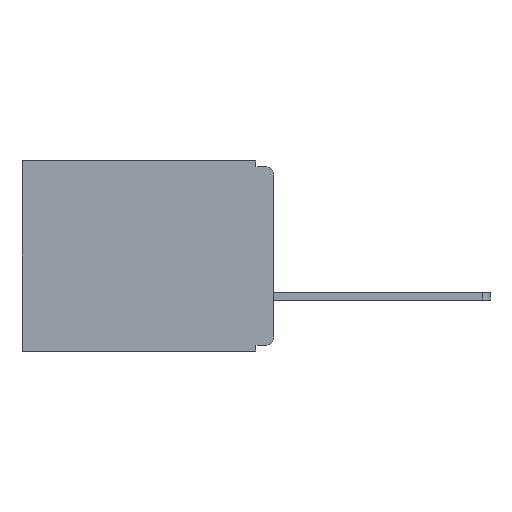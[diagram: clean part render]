
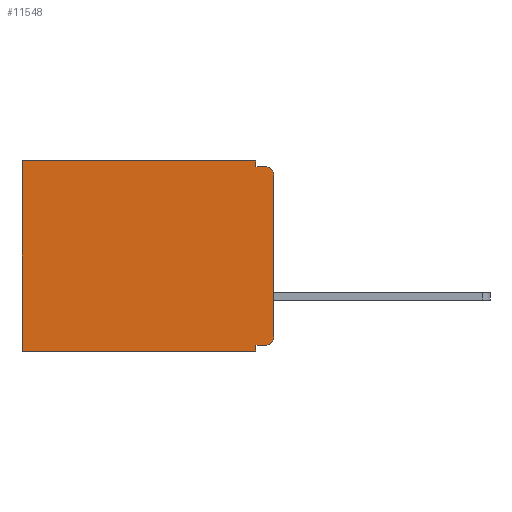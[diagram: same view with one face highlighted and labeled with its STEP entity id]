
A CAD part, left-side view. The second image highlights one B-rep face of the part: STEP entity #11548.
In plain terms, the highlighted planar face has unit normal (-1, 0, 0).
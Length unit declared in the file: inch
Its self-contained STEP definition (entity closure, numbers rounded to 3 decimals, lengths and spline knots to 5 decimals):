
#382 = PLANE ( 'NONE',  #22130 ) ;
#691 = FACE_OUTER_BOUND ( 'NONE', #16390, .T. ) ;
#805 = EDGE_CURVE ( 'NONE', #21169, #20329, #17442, .T. ) ;
#947 = AXIS2_PLACEMENT_3D ( 'NONE', #15070, #13801, #13938 ) ;
#1117 = ORIENTED_EDGE ( 'NONE', *, *, #18474, .T. ) ;
#1120 = CARTESIAN_POINT ( 'NONE',  ( 0.3, 0., -0.305 ) ) ;
#1139 = ORIENTED_EDGE ( 'NONE', *, *, #21667, .F. ) ;
#1445 = ORIENTED_EDGE ( 'NONE', *, *, #17703, .F. ) ;
#1718 = LINE ( 'NONE', #23067, #14266 ) ;
#2388 = EDGE_CURVE ( 'NONE', #6263, #18322, #1718, .T. ) ;
#2704 = VERTEX_POINT ( 'NONE', #6338 ) ;
#2786 = VERTEX_POINT ( 'NONE', #14376 ) ;
#2806 = ORIENTED_EDGE ( 'NONE', *, *, #15526, .F. ) ;
#2977 = VERTEX_POINT ( 'NONE', #6956 ) ;
#3060 = CARTESIAN_POINT ( 'NONE',  ( 0.3, 0.031, -0.33 ) ) ;
#3340 = CARTESIAN_POINT ( 'NONE',  ( 0.3, 0.031, 0. ) ) ;
#3446 = VECTOR ( 'NONE', #3629, 39.37008 ) ;
#3629 = DIRECTION ( 'NONE',  ( 0., -1., 0. ) ) ;
#3724 = CARTESIAN_POINT ( 'NONE',  ( 0.3, 0., -0.32 ) ) ;
#3905 = CARTESIAN_POINT ( 'NONE',  ( 0.3, 0.031, 0. ) ) ;
#4052 = VECTOR ( 'NONE', #10345, 39.37008 ) ;
#4413 = ORIENTED_EDGE ( 'NONE', *, *, #4989, .T. ) ;
#4872 = DIRECTION ( 'NONE',  ( 0., 0., -1. ) ) ;
#4885 = EDGE_CURVE ( 'NONE', #20101, #18322, #5754, .T. ) ;
#4989 = EDGE_CURVE ( 'NONE', #6263, #21406, #13605, .T. ) ;
#5138 = CARTESIAN_POINT ( 'NONE',  ( 0.3, 0.031, -0.01 ) ) ;
#5419 = EDGE_CURVE ( 'NONE', #21169, #2786, #13583, .T. ) ;
#5556 = LINE ( 'NONE', #3724, #14478 ) ;
#5736 = DIRECTION ( 'NONE',  ( 0., 0., -1. ) ) ;
#5754 = CIRCLE ( 'NONE', #947, 0.015 ) ;
#6263 = VERTEX_POINT ( 'NONE', #19391 ) ;
#6317 = LINE ( 'NONE', #3060, #15261 ) ;
#6338 = CARTESIAN_POINT ( 'NONE',  ( 0.3, 0.031, -0.32 ) ) ;
#6956 = CARTESIAN_POINT ( 'NONE',  ( 0.3, 0.031, -0.33 ) ) ;
#8545 = LINE ( 'NONE', #15826, #17480 ) ;
#9005 = DIRECTION ( 'NONE',  ( 0., 1., 0. ) ) ;
#9316 = AXIS2_PLACEMENT_3D ( 'NONE', #11454, #11481, #23077 ) ;
#10345 = DIRECTION ( 'NONE',  ( 0., 1., 0. ) ) ;
#11096 = CARTESIAN_POINT ( 'NONE',  ( 0.3, 0., -0.33 ) ) ;
#11444 = EDGE_CURVE ( 'NONE', #20329, #21406, #22985, .T. ) ;
#11454 = CARTESIAN_POINT ( 'NONE',  ( 0.3, 0.015, -0.025 ) ) ;
#11481 = DIRECTION ( 'NONE',  ( -1., 0., 0. ) ) ;
#11548 = ADVANCED_FACE ( 'NONE', ( #691 ), #382, .F. ) ;
#13583 = LINE ( 'NONE', #14687, #4052 ) ;
#13605 = CIRCLE ( 'NONE', #9316, 0.015 ) ;
#13801 = DIRECTION ( 'NONE',  ( -1., 0., 0. ) ) ;
#13810 = LINE ( 'NONE', #19661, #22700 ) ;
#13938 = DIRECTION ( 'NONE',  ( 0., 0., -1. ) ) ;
#14266 = VECTOR ( 'NONE', #21473, 39.37008 ) ;
#14376 = CARTESIAN_POINT ( 'NONE',  ( 0.3, 0.437, 0. ) ) ;
#14419 = DIRECTION ( 'NONE',  ( 0., 1., 0. ) ) ;
#14478 = VECTOR ( 'NONE', #14419, 39.37008 ) ;
#14687 = CARTESIAN_POINT ( 'NONE',  ( 0.3, 0., 0. ) ) ;
#14897 = DIRECTION ( 'NONE',  ( 0., 0., -1. ) ) ;
#15070 = CARTESIAN_POINT ( 'NONE',  ( 0.3, 0.015, -0.305 ) ) ;
#15261 = VECTOR ( 'NONE', #4872, 39.37008 ) ;
#15526 = EDGE_CURVE ( 'NONE', #20101, #2704, #5556, .T. ) ;
#15826 = CARTESIAN_POINT ( 'NONE',  ( 0.3, 0.437, -0.33 ) ) ;
#16390 = EDGE_LOOP ( 'NONE', ( #18938, #4413, #17535, #22543, #19800, #1117, #1139, #1445, #2806, #22060 ) ) ;
#16435 = DIRECTION ( 'NONE',  ( 1., 0., 0. ) ) ;
#16878 = VECTOR ( 'NONE', #14897, 39.37008 ) ;
#17182 = VERTEX_POINT ( 'NONE', #17537 ) ;
#17442 = LINE ( 'NONE', #3340, #16878 ) ;
#17480 = VECTOR ( 'NONE', #17630, 39.37008 ) ;
#17535 = ORIENTED_EDGE ( 'NONE', *, *, #11444, .F. ) ;
#17537 = CARTESIAN_POINT ( 'NONE',  ( 0.3, 0.437, -0.33 ) ) ;
#17630 = DIRECTION ( 'NONE',  ( 0., 0., -1. ) ) ;
#17703 = EDGE_CURVE ( 'NONE', #2704, #2977, #6317, .T. ) ;
#17928 = CARTESIAN_POINT ( 'NONE',  ( 0.3, 0., -0.01 ) ) ;
#18322 = VERTEX_POINT ( 'NONE', #1120 ) ;
#18474 = EDGE_CURVE ( 'NONE', #2786, #17182, #8545, .T. ) ;
#18758 = CARTESIAN_POINT ( 'NONE',  ( 0.3, 0.015, -0.32 ) ) ;
#18921 = CARTESIAN_POINT ( 'NONE',  ( 0.3, 0.015, -0.01 ) ) ;
#18938 = ORIENTED_EDGE ( 'NONE', *, *, #2388, .F. ) ;
#19391 = CARTESIAN_POINT ( 'NONE',  ( 0.3, 0., -0.025 ) ) ;
#19661 = CARTESIAN_POINT ( 'NONE',  ( 0.3, 0., -0.33 ) ) ;
#19800 = ORIENTED_EDGE ( 'NONE', *, *, #5419, .T. ) ;
#20101 = VERTEX_POINT ( 'NONE', #18758 ) ;
#20329 = VERTEX_POINT ( 'NONE', #5138 ) ;
#21169 = VERTEX_POINT ( 'NONE', #3905 ) ;
#21406 = VERTEX_POINT ( 'NONE', #18921 ) ;
#21473 = DIRECTION ( 'NONE',  ( 0., 0., -1. ) ) ;
#21667 = EDGE_CURVE ( 'NONE', #2977, #17182, #13810, .T. ) ;
#22060 = ORIENTED_EDGE ( 'NONE', *, *, #4885, .T. ) ;
#22130 = AXIS2_PLACEMENT_3D ( 'NONE', #11096, #16435, #5736 ) ;
#22543 = ORIENTED_EDGE ( 'NONE', *, *, #805, .F. ) ;
#22700 = VECTOR ( 'NONE', #9005, 39.37008 ) ;
#22985 = LINE ( 'NONE', #17928, #3446 ) ;
#23067 = CARTESIAN_POINT ( 'NONE',  ( 0.3, 0., -0.33 ) ) ;
#23077 = DIRECTION ( 'NONE',  ( 0., 0., -1. ) ) ;
